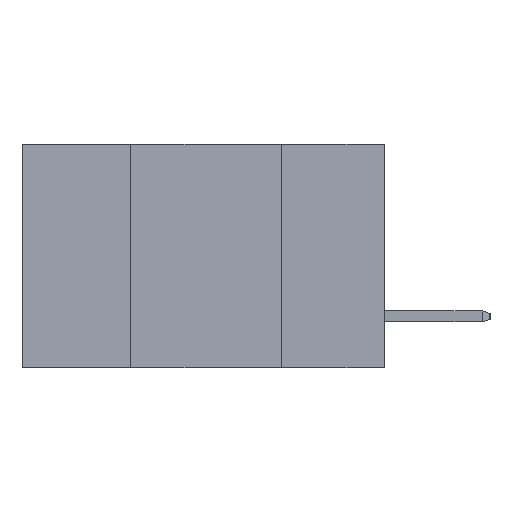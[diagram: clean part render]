
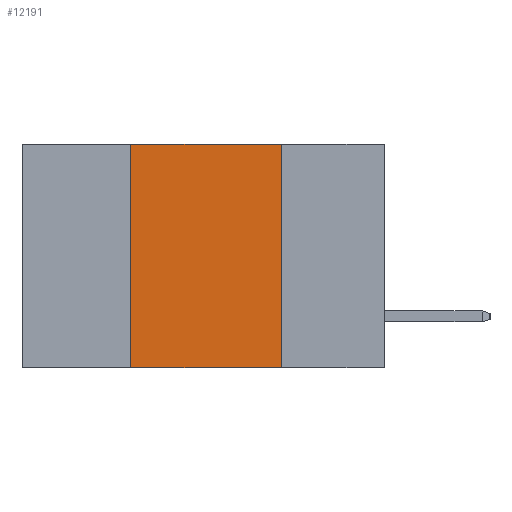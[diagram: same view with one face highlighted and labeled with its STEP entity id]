
A CAD part, left-side view. The second image highlights one B-rep face of the part: STEP entity #12191.
In plain terms, the highlighted planar face has unit normal (-1, 0, 0).
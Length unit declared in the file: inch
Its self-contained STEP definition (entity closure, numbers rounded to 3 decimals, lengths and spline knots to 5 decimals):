
#1265 = EDGE_CURVE ( 'NONE', #3778, #17774, #13418, .T. ) ;
#2982 = DIRECTION ( 'NONE',  ( 0., 0., -1. ) ) ;
#3778 = VERTEX_POINT ( 'NONE', #5748 ) ;
#4098 = PLANE ( 'NONE',  #15301 ) ;
#4243 = VERTEX_POINT ( 'NONE', #14545 ) ;
#5273 = ORIENTED_EDGE ( 'NONE', *, *, #9072, .F. ) ;
#5466 = CARTESIAN_POINT ( 'NONE',  ( 0., 0.42, 0. ) ) ;
#5748 = CARTESIAN_POINT ( 'NONE',  ( 0., 0.42, -0.37 ) ) ;
#7230 = LINE ( 'NONE', #5466, #11959 ) ;
#7442 = LINE ( 'NONE', #15327, #16917 ) ;
#7594 = CARTESIAN_POINT ( 'NONE',  ( 0., 0.6, 0. ) ) ;
#8023 = EDGE_CURVE ( 'NONE', #3778, #4243, #7230, .T. ) ;
#8504 = DIRECTION ( 'NONE',  ( 0., -1., 0. ) ) ;
#8758 = VERTEX_POINT ( 'NONE', #21432 ) ;
#8805 = VECTOR ( 'NONE', #16999, 39.37008 ) ;
#9072 = EDGE_CURVE ( 'NONE', #8758, #17774, #7442, .T. ) ;
#9385 = DIRECTION ( 'NONE',  ( 1., 0., 0. ) ) ;
#9614 = EDGE_CURVE ( 'NONE', #4243, #8758, #17658, .T. ) ;
#9952 = CARTESIAN_POINT ( 'NONE',  ( 0., 0.17, -0.37 ) ) ;
#10976 = CARTESIAN_POINT ( 'NONE',  ( 0., 0.6, -0.37 ) ) ;
#10998 = ORIENTED_EDGE ( 'NONE', *, *, #1265, .T. ) ;
#11624 = ORIENTED_EDGE ( 'NONE', *, *, #8023, .F. ) ;
#11959 = VECTOR ( 'NONE', #17847, 39.37008 ) ;
#12191 = ADVANCED_FACE ( 'NONE', ( #22741 ), #4098, .F. ) ;
#13418 = LINE ( 'NONE', #10976, #22198 ) ;
#14545 = CARTESIAN_POINT ( 'NONE',  ( 0., 0.42, 0. ) ) ;
#15301 = AXIS2_PLACEMENT_3D ( 'NONE', #7594, #9385, #21688 ) ;
#15327 = CARTESIAN_POINT ( 'NONE',  ( 0., 0.17, 0. ) ) ;
#16917 = VECTOR ( 'NONE', #2982, 39.37008 ) ;
#16999 = DIRECTION ( 'NONE',  ( 0., -1., 0. ) ) ;
#17658 = LINE ( 'NONE', #18743, #8805 ) ;
#17774 = VERTEX_POINT ( 'NONE', #9952 ) ;
#17847 = DIRECTION ( 'NONE',  ( 0., 0., 1. ) ) ;
#18743 = CARTESIAN_POINT ( 'NONE',  ( 0., 0.6, 0. ) ) ;
#20435 = ORIENTED_EDGE ( 'NONE', *, *, #9614, .F. ) ;
#21216 = EDGE_LOOP ( 'NONE', ( #5273, #20435, #11624, #10998 ) ) ;
#21432 = CARTESIAN_POINT ( 'NONE',  ( 0., 0.17, 0. ) ) ;
#21688 = DIRECTION ( 'NONE',  ( 0., 0., -1. ) ) ;
#22198 = VECTOR ( 'NONE', #8504, 39.37008 ) ;
#22741 = FACE_OUTER_BOUND ( 'NONE', #21216, .T. ) ;
